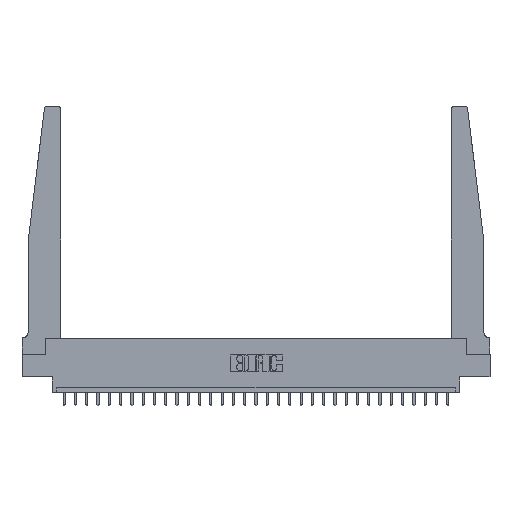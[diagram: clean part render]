
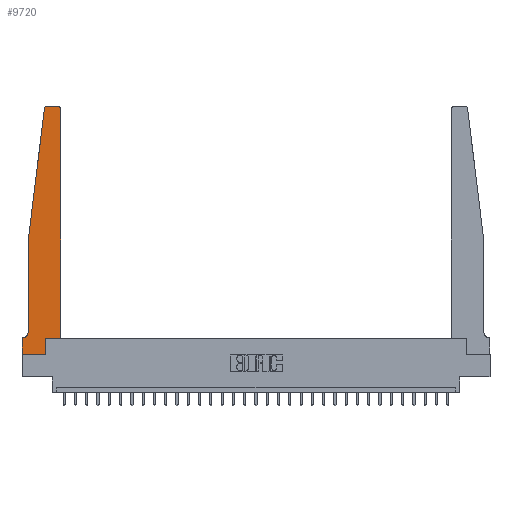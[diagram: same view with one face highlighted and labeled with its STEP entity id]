
A CAD part, top view. The second image highlights one B-rep face of the part: STEP entity #9720.
In plain terms, the highlighted planar face has unit normal (0, 0, 1).
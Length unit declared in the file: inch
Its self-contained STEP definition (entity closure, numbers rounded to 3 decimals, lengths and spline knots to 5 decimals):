
#198 = LINE ( 'NONE', #24256, #5999 ) ;
#227 = VERTEX_POINT ( 'NONE', #3410 ) ;
#380 = LINE ( 'NONE', #9165, #10319 ) ;
#420 = ORIENTED_EDGE ( 'NONE', *, *, #15614, .T. ) ;
#488 = VECTOR ( 'NONE', #2120, 39.37008 ) ;
#662 = CARTESIAN_POINT ( 'NONE',  ( 0.25, 2.75, 0.37 ) ) ;
#1045 = ORIENTED_EDGE ( 'NONE', *, *, #5846, .T. ) ;
#2120 = DIRECTION ( 'NONE',  ( -1., 0., 0. ) ) ;
#2295 = VECTOR ( 'NONE', #18933, 39.37008 ) ;
#2554 = EDGE_CURVE ( 'NONE', #10638, #13357, #11787, .T. ) ;
#2881 = ORIENTED_EDGE ( 'NONE', *, *, #18262, .T. ) ;
#3299 = ORIENTED_EDGE ( 'NONE', *, *, #16955, .T. ) ;
#3373 = LINE ( 'NONE', #23208, #2295 ) ;
#3410 = CARTESIAN_POINT ( 'NONE',  ( 0.395, 2.75, 0.37 ) ) ;
#3673 = DIRECTION ( 'NONE',  ( 1., 0., 0. ) ) ;
#4098 = PLANE ( 'NONE',  #27073 ) ;
#4114 = CARTESIAN_POINT ( 'NONE',  ( 0., 0.1875, 0.37 ) ) ;
#4426 = CARTESIAN_POINT ( 'NONE',  ( 0.425, 0.18, 0.37 ) ) ;
#4607 = CARTESIAN_POINT ( 'NONE',  ( 0.27653, 2.72, 0.37 ) ) ;
#4767 = DIRECTION ( 'NONE',  ( 0., 1., 0. ) ) ;
#5846 = EDGE_CURVE ( 'NONE', #25178, #17957, #380, .T. ) ;
#5958 = DIRECTION ( 'NONE',  ( 0., 0., 1. ) ) ;
#5999 = VECTOR ( 'NONE', #26261, 39.37008 ) ;
#6515 = CARTESIAN_POINT ( 'NONE',  ( 0., 0., 0.37 ) ) ;
#6883 = CARTESIAN_POINT ( 'NONE',  ( 0., 0., 0.37 ) ) ;
#7372 = VERTEX_POINT ( 'NONE', #16931 ) ;
#7583 = ORIENTED_EDGE ( 'NONE', *, *, #26279, .T. ) ;
#7928 = CARTESIAN_POINT ( 'NONE',  ( 0., 0., 0.37 ) ) ;
#8348 = EDGE_CURVE ( 'NONE', #17957, #13729, #23215, .T. ) ;
#9165 = CARTESIAN_POINT ( 'NONE',  ( 0.2605, 0.18, 0.37 ) ) ;
#9720 = ADVANCED_FACE ( 'NONE', ( #12894 ), #4098, .T. ) ;
#10018 = VECTOR ( 'NONE', #22743, 39.37008 ) ;
#10301 = CARTESIAN_POINT ( 'NONE',  ( 0.065, 1.25, 0.37 ) ) ;
#10319 = VECTOR ( 'NONE', #4767, 39.37008 ) ;
#10371 = DIRECTION ( 'NONE',  ( 1., 0., 0. ) ) ;
#10638 = VERTEX_POINT ( 'NONE', #12680 ) ;
#10858 = DIRECTION ( 'NONE',  ( 1., 0., 0. ) ) ;
#10917 = ORIENTED_EDGE ( 'NONE', *, *, #27878, .T. ) ;
#11101 = LINE ( 'NONE', #4426, #27098 ) ;
#11679 = EDGE_LOOP ( 'NONE', ( #3299, #7583, #17376, #18084, #16836, #10917, #2881, #420, #1045, #15265, #23533, #27011 ) ) ;
#11787 = CIRCLE ( 'NONE', #19016, 0.05 ) ;
#12301 = VERTEX_POINT ( 'NONE', #7928 ) ;
#12680 = CARTESIAN_POINT ( 'NONE',  ( 0.065, 0.2375, 0.37 ) ) ;
#12754 = DIRECTION ( 'NONE',  ( 0., 0., 1. ) ) ;
#12878 = CARTESIAN_POINT ( 'NONE',  ( 0.425, 2.72, 0.37 ) ) ;
#12894 = FACE_OUTER_BOUND ( 'NONE', #11679, .T. ) ;
#12962 = EDGE_CURVE ( 'NONE', #13729, #24687, #11101, .T. ) ;
#13120 = VERTEX_POINT ( 'NONE', #25515 ) ;
#13321 = DIRECTION ( 'NONE',  ( 0., -1., 0. ) ) ;
#13357 = VERTEX_POINT ( 'NONE', #23804 ) ;
#13729 = VERTEX_POINT ( 'NONE', #26330 ) ;
#14125 = LINE ( 'NONE', #10301, #10018 ) ;
#14581 = AXIS2_PLACEMENT_3D ( 'NONE', #14765, #5958, #10371 ) ;
#14765 = CARTESIAN_POINT ( 'NONE',  ( 0.395, 2.72, 0.37 ) ) ;
#14826 = DIRECTION ( 'NONE',  ( 0., 0., 1. ) ) ;
#14979 = VECTOR ( 'NONE', #22171, 39.37008 ) ;
#15016 = DIRECTION ( 'NONE',  ( 1., 0., 0. ) ) ;
#15022 = LINE ( 'NONE', #662, #488 ) ;
#15265 = ORIENTED_EDGE ( 'NONE', *, *, #8348, .T. ) ;
#15614 = EDGE_CURVE ( 'NONE', #12301, #25178, #21760, .T. ) ;
#16836 = ORIENTED_EDGE ( 'NONE', *, *, #2554, .T. ) ;
#16931 = CARTESIAN_POINT ( 'NONE',  ( 0.24675, 2.72367, 0.37 ) ) ;
#16955 = EDGE_CURVE ( 'NONE', #227, #25214, #15022, .T. ) ;
#17376 = ORIENTED_EDGE ( 'NONE', *, *, #25782, .T. ) ;
#17753 = CARTESIAN_POINT ( 'NONE',  ( 0.27653, 2.75, 0.37 ) ) ;
#17957 = VERTEX_POINT ( 'NONE', #20123 ) ;
#18084 = ORIENTED_EDGE ( 'NONE', *, *, #26059, .T. ) ;
#18262 = EDGE_CURVE ( 'NONE', #24177, #12301, #26218, .T. ) ;
#18933 = DIRECTION ( 'NONE',  ( -0.122, -0.992, 0. ) ) ;
#19016 = AXIS2_PLACEMENT_3D ( 'NONE', #19734, #24125, #19865 ) ;
#19251 = VECTOR ( 'NONE', #3673, 39.37008 ) ;
#19513 = AXIS2_PLACEMENT_3D ( 'NONE', #4607, #14826, #10858 ) ;
#19727 = DIRECTION ( 'NONE',  ( 0., 1., 0. ) ) ;
#19734 = CARTESIAN_POINT ( 'NONE',  ( 0.015, 0.2375, 0.37 ) ) ;
#19865 = DIRECTION ( 'NONE',  ( -1., 0., 0. ) ) ;
#20123 = CARTESIAN_POINT ( 'NONE',  ( 0.2605, 0.18, 0.37 ) ) ;
#20395 = CIRCLE ( 'NONE', #19513, 0.03 ) ;
#21336 = VECTOR ( 'NONE', #13321, 39.37008 ) ;
#21647 = CARTESIAN_POINT ( 'NONE',  ( 0., 0.1875, 0.37 ) ) ;
#21760 = LINE ( 'NONE', #6883, #14979 ) ;
#21878 = CARTESIAN_POINT ( 'NONE',  ( 0.2605, 0., 0.37 ) ) ;
#22171 = DIRECTION ( 'NONE',  ( 1., 0., 0. ) ) ;
#22743 = DIRECTION ( 'NONE',  ( 0., -1., 0. ) ) ;
#23162 = CIRCLE ( 'NONE', #14581, 0.03 ) ;
#23208 = CARTESIAN_POINT ( 'NONE',  ( 0.065, 1.25, 0.37 ) ) ;
#23215 = LINE ( 'NONE', #25487, #19251 ) ;
#23533 = ORIENTED_EDGE ( 'NONE', *, *, #12962, .T. ) ;
#23804 = CARTESIAN_POINT ( 'NONE',  ( 0.015, 0.1875, 0.37 ) ) ;
#24125 = DIRECTION ( 'NONE',  ( 0., 0., -1. ) ) ;
#24177 = VERTEX_POINT ( 'NONE', #4114 ) ;
#24256 = CARTESIAN_POINT ( 'NONE',  ( 0.065, 0.1875, 0.37 ) ) ;
#24687 = VERTEX_POINT ( 'NONE', #12878 ) ;
#25178 = VERTEX_POINT ( 'NONE', #21878 ) ;
#25214 = VERTEX_POINT ( 'NONE', #17753 ) ;
#25487 = CARTESIAN_POINT ( 'NONE',  ( 0.425, 0.18, 0.37 ) ) ;
#25515 = CARTESIAN_POINT ( 'NONE',  ( 0.065, 1.25, 0.37 ) ) ;
#25782 = EDGE_CURVE ( 'NONE', #7372, #13120, #3373, .T. ) ;
#26059 = EDGE_CURVE ( 'NONE', #13120, #10638, #14125, .T. ) ;
#26218 = LINE ( 'NONE', #6515, #21336 ) ;
#26261 = DIRECTION ( 'NONE',  ( -1., 0., 0. ) ) ;
#26279 = EDGE_CURVE ( 'NONE', #25214, #7372, #20395, .T. ) ;
#26330 = CARTESIAN_POINT ( 'NONE',  ( 0.425, 0.18, 0.37 ) ) ;
#27011 = ORIENTED_EDGE ( 'NONE', *, *, #27041, .T. ) ;
#27041 = EDGE_CURVE ( 'NONE', #24687, #227, #23162, .T. ) ;
#27073 = AXIS2_PLACEMENT_3D ( 'NONE', #21647, #12754, #15016 ) ;
#27098 = VECTOR ( 'NONE', #19727, 39.37008 ) ;
#27878 = EDGE_CURVE ( 'NONE', #13357, #24177, #198, .T. ) ;
